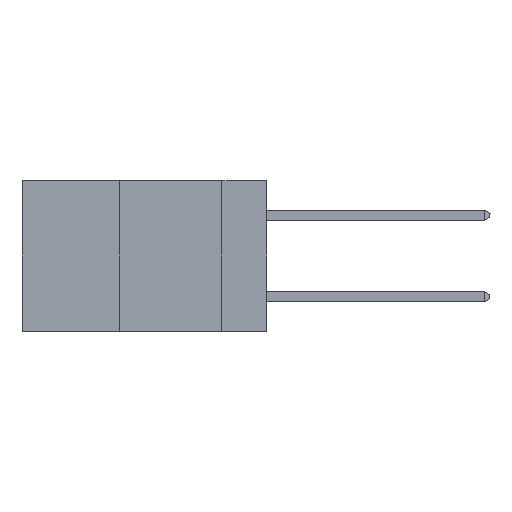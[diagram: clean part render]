
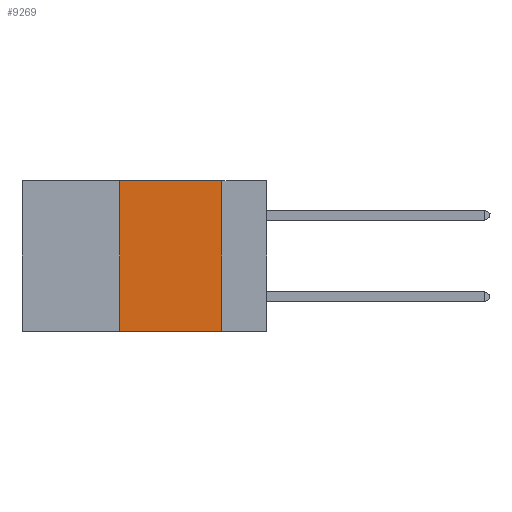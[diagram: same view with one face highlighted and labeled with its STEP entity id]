
A CAD part, left-side view. The second image highlights one B-rep face of the part: STEP entity #9269.
In plain terms, the highlighted planar face has unit normal (-1, 0, 0).
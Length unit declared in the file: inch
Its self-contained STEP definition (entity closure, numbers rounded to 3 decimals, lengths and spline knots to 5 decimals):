
#294 = CARTESIAN_POINT ( 'NONE',  ( 0., 0.11, -0.37 ) ) ;
#761 = EDGE_CURVE ( 'NONE', #18461, #9497, #16062, .T. ) ;
#1148 = VECTOR ( 'NONE', #24359, 39.37008 ) ;
#1320 = DIRECTION ( 'NONE',  ( 0., -1., 0. ) ) ;
#3033 = ORIENTED_EDGE ( 'NONE', *, *, #23096, .F. ) ;
#3283 = DIRECTION ( 'NONE',  ( 1., 0., 0. ) ) ;
#6491 = CARTESIAN_POINT ( 'NONE',  ( 0., 0.36, 0. ) ) ;
#6631 = EDGE_CURVE ( 'NONE', #17671, #9497, #8708, .T. ) ;
#6704 = EDGE_CURVE ( 'NONE', #21213, #17671, #6870, .T. ) ;
#6795 = VECTOR ( 'NONE', #8283, 39.37008 ) ;
#6870 = LINE ( 'NONE', #21867, #19735 ) ;
#8283 = DIRECTION ( 'NONE',  ( 0., 0., 1. ) ) ;
#8517 = EDGE_LOOP ( 'NONE', ( #16764, #15544, #3033, #19531 ) ) ;
#8622 = LINE ( 'NONE', #6491, #6795 ) ;
#8708 = LINE ( 'NONE', #22560, #11433 ) ;
#9269 = ADVANCED_FACE ( 'NONE', ( #9412 ), #17180, .F. ) ;
#9412 = FACE_OUTER_BOUND ( 'NONE', #8517, .T. ) ;
#9497 = VERTEX_POINT ( 'NONE', #294 ) ;
#10758 = DIRECTION ( 'NONE',  ( 0., 0., -1. ) ) ;
#11055 = AXIS2_PLACEMENT_3D ( 'NONE', #14930, #3283, #18880 ) ;
#11433 = VECTOR ( 'NONE', #10758, 39.37008 ) ;
#14930 = CARTESIAN_POINT ( 'NONE',  ( 0., 0.6, 0. ) ) ;
#15544 = ORIENTED_EDGE ( 'NONE', *, *, #6704, .F. ) ;
#15634 = CARTESIAN_POINT ( 'NONE',  ( 0., 0.11, 0. ) ) ;
#16062 = LINE ( 'NONE', #18300, #1148 ) ;
#16764 = ORIENTED_EDGE ( 'NONE', *, *, #6631, .F. ) ;
#17180 = PLANE ( 'NONE',  #11055 ) ;
#17671 = VERTEX_POINT ( 'NONE', #15634 ) ;
#18300 = CARTESIAN_POINT ( 'NONE',  ( 0., 0.6, -0.37 ) ) ;
#18461 = VERTEX_POINT ( 'NONE', #19727 ) ;
#18880 = DIRECTION ( 'NONE',  ( 0., 0., -1. ) ) ;
#19531 = ORIENTED_EDGE ( 'NONE', *, *, #761, .T. ) ;
#19727 = CARTESIAN_POINT ( 'NONE',  ( 0., 0.36, -0.37 ) ) ;
#19735 = VECTOR ( 'NONE', #1320, 39.37008 ) ;
#21213 = VERTEX_POINT ( 'NONE', #22163 ) ;
#21867 = CARTESIAN_POINT ( 'NONE',  ( 0., 0.6, 0. ) ) ;
#22163 = CARTESIAN_POINT ( 'NONE',  ( 0., 0.36, 0. ) ) ;
#22560 = CARTESIAN_POINT ( 'NONE',  ( 0., 0.11, 0. ) ) ;
#23096 = EDGE_CURVE ( 'NONE', #18461, #21213, #8622, .T. ) ;
#24359 = DIRECTION ( 'NONE',  ( 0., -1., 0. ) ) ;
